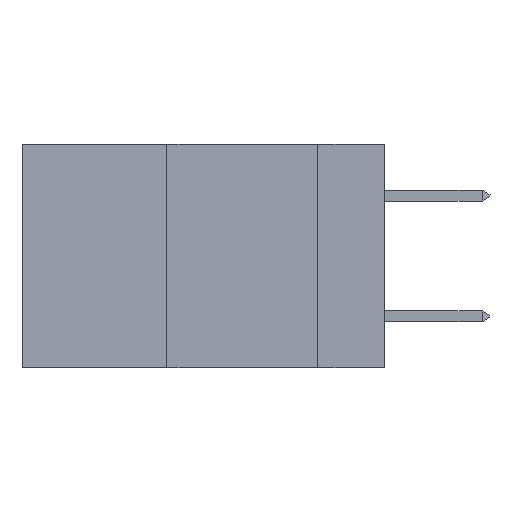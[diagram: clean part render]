
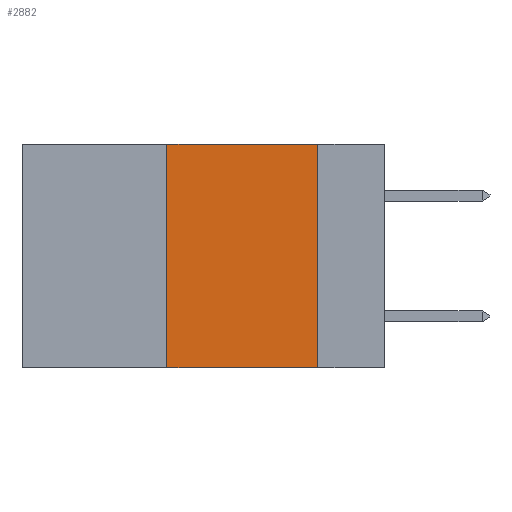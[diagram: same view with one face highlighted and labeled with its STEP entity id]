
A CAD part, left-side view. The second image highlights one B-rep face of the part: STEP entity #2882.
In plain terms, the highlighted planar face has unit normal (-1, 0, 0).
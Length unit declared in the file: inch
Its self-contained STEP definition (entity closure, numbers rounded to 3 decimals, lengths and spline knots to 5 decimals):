
#242 = LINE ( 'NONE', #5530, #7431 ) ;
#1097 = DIRECTION ( 'NONE',  ( 0., 0., -1. ) ) ;
#1214 = DIRECTION ( 'NONE',  ( 0., -1., 0. ) ) ;
#1263 = VECTOR ( 'NONE', #7927, 39.37008 ) ;
#1271 = PLANE ( 'NONE',  #9927 ) ;
#1643 = VERTEX_POINT ( 'NONE', #10515 ) ;
#1684 = ORIENTED_EDGE ( 'NONE', *, *, #6999, .F. ) ;
#1843 = VECTOR ( 'NONE', #5263, 39.37008 ) ;
#1930 = CARTESIAN_POINT ( 'NONE',  ( 0., 0.36, 0. ) ) ;
#1951 = ORIENTED_EDGE ( 'NONE', *, *, #3904, .T. ) ;
#2487 = CARTESIAN_POINT ( 'NONE',  ( 0., 0.11, -0.37 ) ) ;
#2882 = ADVANCED_FACE ( 'NONE', ( #9094 ), #1271, .F. ) ;
#2973 = DIRECTION ( 'NONE',  ( 0., 0., -1. ) ) ;
#3866 = LINE ( 'NONE', #1930, #1263 ) ;
#3904 = EDGE_CURVE ( 'NONE', #10453, #5152, #10832, .T. ) ;
#5152 = VERTEX_POINT ( 'NONE', #2487 ) ;
#5263 = DIRECTION ( 'NONE',  ( 0., -1., 0. ) ) ;
#5387 = CARTESIAN_POINT ( 'NONE',  ( 0., 0.36, -0.37 ) ) ;
#5530 = CARTESIAN_POINT ( 'NONE',  ( 0., 0.6, 0. ) ) ;
#6941 = EDGE_CURVE ( 'NONE', #10453, #1643, #3866, .T. ) ;
#6999 = EDGE_CURVE ( 'NONE', #10233, #5152, #9777, .T. ) ;
#7356 = VECTOR ( 'NONE', #1097, 39.37008 ) ;
#7431 = VECTOR ( 'NONE', #1214, 39.37008 ) ;
#7812 = CARTESIAN_POINT ( 'NONE',  ( 0., 0.6, -0.37 ) ) ;
#7927 = DIRECTION ( 'NONE',  ( 0., 0., 1. ) ) ;
#8132 = CARTESIAN_POINT ( 'NONE',  ( 0., 0.6, 0. ) ) ;
#8162 = DIRECTION ( 'NONE',  ( 1., 0., 0. ) ) ;
#8546 = ORIENTED_EDGE ( 'NONE', *, *, #9121, .F. ) ;
#9094 = FACE_OUTER_BOUND ( 'NONE', #10708, .T. ) ;
#9121 = EDGE_CURVE ( 'NONE', #1643, #10233, #242, .T. ) ;
#9777 = LINE ( 'NONE', #10409, #7356 ) ;
#9927 = AXIS2_PLACEMENT_3D ( 'NONE', #8132, #8162, #2973 ) ;
#10165 = CARTESIAN_POINT ( 'NONE',  ( 0., 0.11, 0. ) ) ;
#10233 = VERTEX_POINT ( 'NONE', #10165 ) ;
#10409 = CARTESIAN_POINT ( 'NONE',  ( 0., 0.11, 0. ) ) ;
#10453 = VERTEX_POINT ( 'NONE', #5387 ) ;
#10515 = CARTESIAN_POINT ( 'NONE',  ( 0., 0.36, 0. ) ) ;
#10694 = ORIENTED_EDGE ( 'NONE', *, *, #6941, .F. ) ;
#10708 = EDGE_LOOP ( 'NONE', ( #1684, #8546, #10694, #1951 ) ) ;
#10832 = LINE ( 'NONE', #7812, #1843 ) ;
